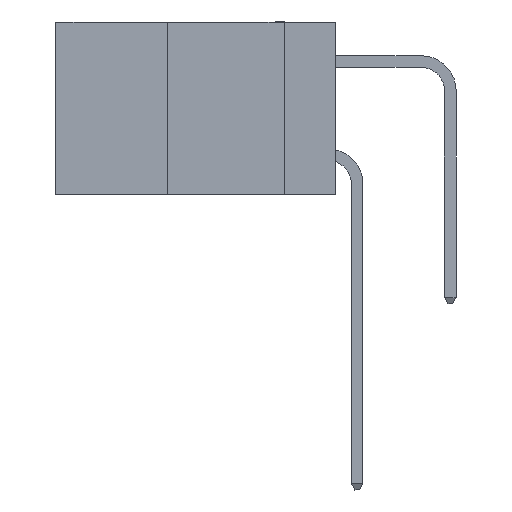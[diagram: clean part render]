
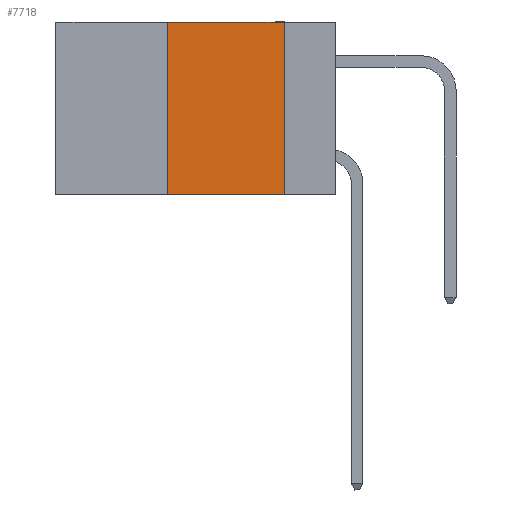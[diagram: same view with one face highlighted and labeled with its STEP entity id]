
A CAD part, left-side view. The second image highlights one B-rep face of the part: STEP entity #7718.
In plain terms, the highlighted planar face has unit normal (-1, 0, 0).
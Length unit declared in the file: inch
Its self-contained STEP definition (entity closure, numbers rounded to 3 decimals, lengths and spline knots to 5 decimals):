
#2467 = DIRECTION ( 'NONE',  ( 0., 0., -1. ) ) ;
#3077 = VERTEX_POINT ( 'NONE', #10860 ) ;
#4312 = VECTOR ( 'NONE', #2467, 39.37008 ) ;
#4572 = AXIS2_PLACEMENT_3D ( 'NONE', #37662, #11465, #31179 ) ;
#6621 = CARTESIAN_POINT ( 'NONE',  ( 0., 0.11, 0. ) ) ;
#6981 = EDGE_CURVE ( 'NONE', #3077, #35270, #25112, .T. ) ;
#7718 = ADVANCED_FACE ( 'NONE', ( #19520 ), #11282, .F. ) ;
#7914 = ORIENTED_EDGE ( 'NONE', *, *, #16644, .F. ) ;
#8587 = CARTESIAN_POINT ( 'NONE',  ( 0., 0.11, 0. ) ) ;
#9675 = LINE ( 'NONE', #24404, #22493 ) ;
#9690 = VERTEX_POINT ( 'NONE', #6621 ) ;
#10860 = CARTESIAN_POINT ( 'NONE',  ( 0., 0.36, -0.37 ) ) ;
#10901 = LINE ( 'NONE', #13773, #36933 ) ;
#11282 = PLANE ( 'NONE',  #4572 ) ;
#11465 = DIRECTION ( 'NONE',  ( 1., 0., 0. ) ) ;
#12111 = EDGE_CURVE ( 'NONE', #16710, #9690, #9675, .T. ) ;
#13773 = CARTESIAN_POINT ( 'NONE',  ( 0., 0.36, 0. ) ) ;
#13996 = CARTESIAN_POINT ( 'NONE',  ( 0., 0.6, -0.37 ) ) ;
#14386 = EDGE_CURVE ( 'NONE', #3077, #16710, #10901, .T. ) ;
#16034 = EDGE_LOOP ( 'NONE', ( #7914, #32314, #33968, #26128 ) ) ;
#16644 = EDGE_CURVE ( 'NONE', #9690, #35270, #28099, .T. ) ;
#16710 = VERTEX_POINT ( 'NONE', #31155 ) ;
#19520 = FACE_OUTER_BOUND ( 'NONE', #16034, .T. ) ;
#22493 = VECTOR ( 'NONE', #24783, 39.37008 ) ;
#22806 = DIRECTION ( 'NONE',  ( 0., -1., 0. ) ) ;
#24404 = CARTESIAN_POINT ( 'NONE',  ( 0., 0.6, 0. ) ) ;
#24783 = DIRECTION ( 'NONE',  ( 0., -1., 0. ) ) ;
#25112 = LINE ( 'NONE', #13996, #35125 ) ;
#26128 = ORIENTED_EDGE ( 'NONE', *, *, #6981, .T. ) ;
#28099 = LINE ( 'NONE', #8587, #4312 ) ;
#29345 = CARTESIAN_POINT ( 'NONE',  ( 0., 0.11, -0.37 ) ) ;
#31155 = CARTESIAN_POINT ( 'NONE',  ( 0., 0.36, 0. ) ) ;
#31179 = DIRECTION ( 'NONE',  ( 0., 0., -1. ) ) ;
#32314 = ORIENTED_EDGE ( 'NONE', *, *, #12111, .F. ) ;
#33968 = ORIENTED_EDGE ( 'NONE', *, *, #14386, .F. ) ;
#35125 = VECTOR ( 'NONE', #22806, 39.37008 ) ;
#35270 = VERTEX_POINT ( 'NONE', #29345 ) ;
#36933 = VECTOR ( 'NONE', #37093, 39.37008 ) ;
#37093 = DIRECTION ( 'NONE',  ( 0., 0., 1. ) ) ;
#37662 = CARTESIAN_POINT ( 'NONE',  ( 0., 0.6, 0. ) ) ;
